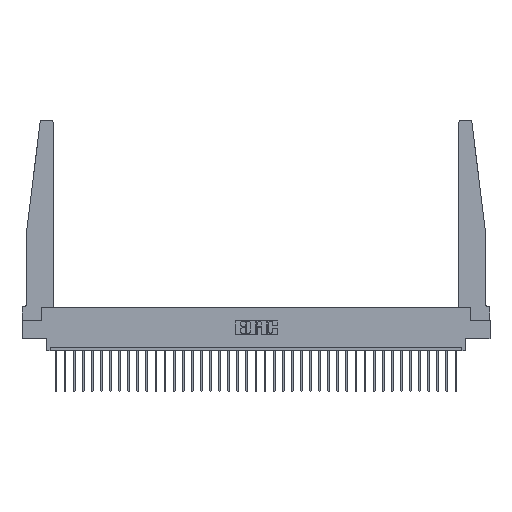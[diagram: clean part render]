
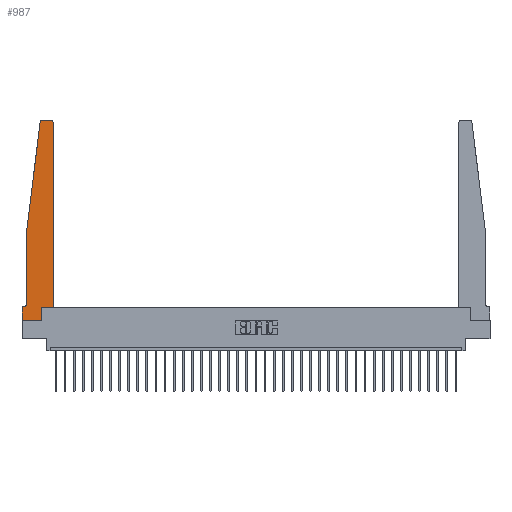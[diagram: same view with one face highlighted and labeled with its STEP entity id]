
A CAD part, top view. The second image highlights one B-rep face of the part: STEP entity #987.
In plain terms, the highlighted planar face has unit normal (0, 0, 1).
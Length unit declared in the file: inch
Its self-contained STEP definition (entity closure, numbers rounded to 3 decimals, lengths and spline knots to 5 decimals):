
#136 = LINE ( 'NONE', #10256, #20693 ) ;
#354 = CARTESIAN_POINT ( 'NONE',  ( 0.065, 1.25, 0.37 ) ) ;
#503 = ORIENTED_EDGE ( 'NONE', *, *, #28427, .T. ) ;
#738 = CARTESIAN_POINT ( 'NONE',  ( 0.27653, 2.75, 0.37 ) ) ;
#837 = CARTESIAN_POINT ( 'NONE',  ( 0., 0., 0.37 ) ) ;
#874 = EDGE_CURVE ( 'NONE', #23549, #18325, #25369, .T. ) ;
#987 = ADVANCED_FACE ( 'NONE', ( #32881 ), #10285, .T. ) ;
#1087 = CARTESIAN_POINT ( 'NONE',  ( 0., 0.1875, 0.37 ) ) ;
#1746 = CARTESIAN_POINT ( 'NONE',  ( 0.015, 0.2375, 0.37 ) ) ;
#2145 = CARTESIAN_POINT ( 'NONE',  ( 0.065, 1.25, 0.37 ) ) ;
#2150 = DIRECTION ( 'NONE',  ( 1., 0., 0. ) ) ;
#2809 = DIRECTION ( 'NONE',  ( 1., 0., 0. ) ) ;
#2934 = DIRECTION ( 'NONE',  ( 0., 1., 0. ) ) ;
#3147 = VERTEX_POINT ( 'NONE', #354 ) ;
#3248 = DIRECTION ( 'NONE',  ( 1., 0., 0. ) ) ;
#4034 = CARTESIAN_POINT ( 'NONE',  ( 0.065, 0.2375, 0.37 ) ) ;
#4301 = VERTEX_POINT ( 'NONE', #1087 ) ;
#4602 = ORIENTED_EDGE ( 'NONE', *, *, #874, .T. ) ;
#4941 = CARTESIAN_POINT ( 'NONE',  ( 0.425, 0.18, 0.37 ) ) ;
#5286 = DIRECTION ( 'NONE',  ( 0., 0., 1. ) ) ;
#5468 = VERTEX_POINT ( 'NONE', #31527 ) ;
#6330 = EDGE_LOOP ( 'NONE', ( #29608, #23173, #503, #9494, #22351, #10316, #22967, #32261, #27560, #23939, #12978, #4602 ) ) ;
#6825 = EDGE_CURVE ( 'NONE', #5468, #7841, #31537, .T. ) ;
#6980 = EDGE_CURVE ( 'NONE', #27226, #23549, #29550, .T. ) ;
#7213 = DIRECTION ( 'NONE',  ( 0., 1., 0. ) ) ;
#7278 = CARTESIAN_POINT ( 'NONE',  ( 0.395, 2.72, 0.37 ) ) ;
#7393 = VECTOR ( 'NONE', #11584, 39.37008 ) ;
#7788 = VECTOR ( 'NONE', #3248, 39.37008 ) ;
#7841 = VERTEX_POINT ( 'NONE', #31618 ) ;
#9494 = ORIENTED_EDGE ( 'NONE', *, *, #24033, .T. ) ;
#9806 = VERTEX_POINT ( 'NONE', #32227 ) ;
#10119 = CARTESIAN_POINT ( 'NONE',  ( 0., 0.1875, 0.37 ) ) ;
#10256 = CARTESIAN_POINT ( 'NONE',  ( 0.065, 0.1875, 0.37 ) ) ;
#10285 = PLANE ( 'NONE',  #32820 ) ;
#10316 = ORIENTED_EDGE ( 'NONE', *, *, #10594, .T. ) ;
#10594 = EDGE_CURVE ( 'NONE', #9806, #4301, #136, .T. ) ;
#11584 = DIRECTION ( 'NONE',  ( 1., 0., 0. ) ) ;
#12080 = CARTESIAN_POINT ( 'NONE',  ( 0.425, 0.18, 0.37 ) ) ;
#12752 = VECTOR ( 'NONE', #18042, 39.37008 ) ;
#12978 = ORIENTED_EDGE ( 'NONE', *, *, #6980, .T. ) ;
#13008 = AXIS2_PLACEMENT_3D ( 'NONE', #1746, #16211, #24026 ) ;
#13886 = CARTESIAN_POINT ( 'NONE',  ( 0., 0., 0.37 ) ) ;
#14733 = DIRECTION ( 'NONE',  ( -1., 0., 0. ) ) ;
#14952 = EDGE_CURVE ( 'NONE', #20793, #26938, #27700, .T. ) ;
#15537 = CARTESIAN_POINT ( 'NONE',  ( 0.27653, 2.72, 0.37 ) ) ;
#15747 = CARTESIAN_POINT ( 'NONE',  ( 0.2605, 0.18, 0.37 ) ) ;
#16211 = DIRECTION ( 'NONE',  ( 0., 0., -1. ) ) ;
#16460 = DIRECTION ( 'NONE',  ( 0., -1., 0. ) ) ;
#17749 = LINE ( 'NONE', #27895, #20814 ) ;
#18042 = DIRECTION ( 'NONE',  ( 0., -1., 0. ) ) ;
#18088 = VECTOR ( 'NONE', #2934, 39.37008 ) ;
#18250 = LINE ( 'NONE', #31830, #18088 ) ;
#18325 = VERTEX_POINT ( 'NONE', #31548 ) ;
#18571 = EDGE_CURVE ( 'NONE', #18325, #20793, #17749, .T. ) ;
#18959 = LINE ( 'NONE', #837, #27598 ) ;
#19825 = VECTOR ( 'NONE', #20283, 39.37008 ) ;
#20032 = AXIS2_PLACEMENT_3D ( 'NONE', #7278, #25275, #2150 ) ;
#20213 = EDGE_CURVE ( 'NONE', #27565, #9806, #22081, .T. ) ;
#20283 = DIRECTION ( 'NONE',  ( -0.122, -0.992, 0. ) ) ;
#20417 = DIRECTION ( 'NONE',  ( -1., 0., 0. ) ) ;
#20690 = LINE ( 'NONE', #30848, #12752 ) ;
#20693 = VECTOR ( 'NONE', #20417, 39.37008 ) ;
#20793 = VERTEX_POINT ( 'NONE', #738 ) ;
#20814 = VECTOR ( 'NONE', #14733, 39.37008 ) ;
#22081 = CIRCLE ( 'NONE', #13008, 0.05 ) ;
#22218 = CARTESIAN_POINT ( 'NONE',  ( 0.425, 0.18, 0.37 ) ) ;
#22351 = ORIENTED_EDGE ( 'NONE', *, *, #20213, .T. ) ;
#22412 = CARTESIAN_POINT ( 'NONE',  ( 0.425, 2.72, 0.37 ) ) ;
#22952 = EDGE_CURVE ( 'NONE', #4301, #5468, #18959, .T. ) ;
#22967 = ORIENTED_EDGE ( 'NONE', *, *, #22952, .T. ) ;
#23173 = ORIENTED_EDGE ( 'NONE', *, *, #14952, .T. ) ;
#23348 = DIRECTION ( 'NONE',  ( 1., 0., 0. ) ) ;
#23449 = EDGE_CURVE ( 'NONE', #25635, #27226, #29414, .T. ) ;
#23549 = VERTEX_POINT ( 'NONE', #22412 ) ;
#23939 = ORIENTED_EDGE ( 'NONE', *, *, #23449, .T. ) ;
#24026 = DIRECTION ( 'NONE',  ( -1., 0., 0. ) ) ;
#24033 = EDGE_CURVE ( 'NONE', #3147, #27565, #20690, .T. ) ;
#24546 = EDGE_CURVE ( 'NONE', #7841, #25635, #18250, .T. ) ;
#25275 = DIRECTION ( 'NONE',  ( 0., 0., 1. ) ) ;
#25369 = CIRCLE ( 'NONE', #20032, 0.03 ) ;
#25635 = VERTEX_POINT ( 'NONE', #15747 ) ;
#26938 = VERTEX_POINT ( 'NONE', #28450 ) ;
#27226 = VERTEX_POINT ( 'NONE', #4941 ) ;
#27560 = ORIENTED_EDGE ( 'NONE', *, *, #24546, .T. ) ;
#27565 = VERTEX_POINT ( 'NONE', #4034 ) ;
#27598 = VECTOR ( 'NONE', #16460, 39.37008 ) ;
#27700 = CIRCLE ( 'NONE', #29289, 0.03 ) ;
#27873 = DIRECTION ( 'NONE',  ( 0., 0., 1. ) ) ;
#27895 = CARTESIAN_POINT ( 'NONE',  ( 0.25, 2.75, 0.37 ) ) ;
#28427 = EDGE_CURVE ( 'NONE', #26938, #3147, #32597, .T. ) ;
#28450 = CARTESIAN_POINT ( 'NONE',  ( 0.24675, 2.72367, 0.37 ) ) ;
#29289 = AXIS2_PLACEMENT_3D ( 'NONE', #15537, #27873, #23348 ) ;
#29414 = LINE ( 'NONE', #12080, #7393 ) ;
#29541 = VECTOR ( 'NONE', #7213, 39.37008 ) ;
#29550 = LINE ( 'NONE', #22218, #29541 ) ;
#29608 = ORIENTED_EDGE ( 'NONE', *, *, #18571, .T. ) ;
#30848 = CARTESIAN_POINT ( 'NONE',  ( 0.065, 1.25, 0.37 ) ) ;
#31527 = CARTESIAN_POINT ( 'NONE',  ( 0., 0., 0.37 ) ) ;
#31537 = LINE ( 'NONE', #13886, #7788 ) ;
#31548 = CARTESIAN_POINT ( 'NONE',  ( 0.395, 2.75, 0.37 ) ) ;
#31618 = CARTESIAN_POINT ( 'NONE',  ( 0.2605, 0., 0.37 ) ) ;
#31830 = CARTESIAN_POINT ( 'NONE',  ( 0.2605, 0.18, 0.37 ) ) ;
#32227 = CARTESIAN_POINT ( 'NONE',  ( 0.015, 0.1875, 0.37 ) ) ;
#32261 = ORIENTED_EDGE ( 'NONE', *, *, #6825, .T. ) ;
#32597 = LINE ( 'NONE', #2145, #19825 ) ;
#32820 = AXIS2_PLACEMENT_3D ( 'NONE', #10119, #5286, #2809 ) ;
#32881 = FACE_OUTER_BOUND ( 'NONE', #6330, .T. ) ;
